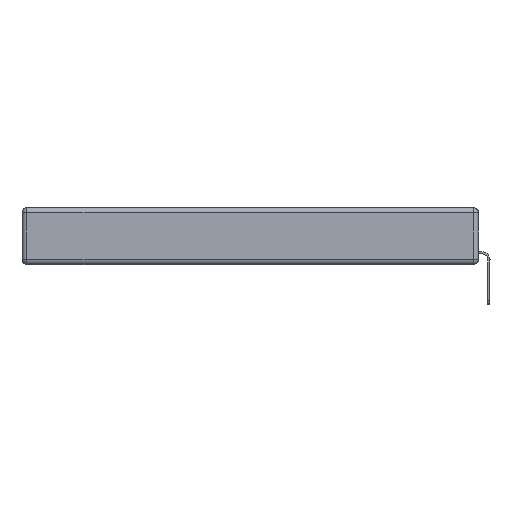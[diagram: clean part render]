
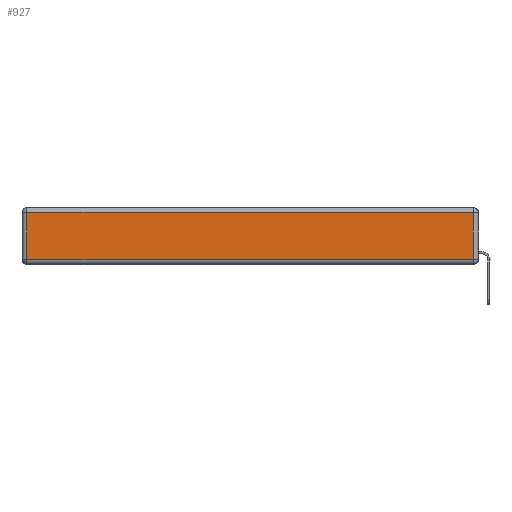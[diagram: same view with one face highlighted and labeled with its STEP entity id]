
A CAD part, left-side view. The second image highlights one B-rep face of the part: STEP entity #927.
In plain terms, the highlighted planar face has unit normal (-1, 0, 0).
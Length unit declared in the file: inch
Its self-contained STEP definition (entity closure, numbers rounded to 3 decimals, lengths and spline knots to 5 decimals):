
#693 = CARTESIAN_POINT ( 'NONE',  ( 0., 0., -0.313 ) ) ;
#814 = DIRECTION ( 'NONE',  ( 0., 0., 1. ) ) ;
#927 = ADVANCED_FACE ( 'NONE', ( #8406 ), #14898, .T. ) ;
#1033 = DIRECTION ( 'NONE',  ( 0., 0., 1. ) ) ;
#1086 = ORIENTED_EDGE ( 'NONE', *, *, #10584, .T. ) ;
#1088 = LINE ( 'NONE', #16699, #4471 ) ;
#1699 = AXIS2_PLACEMENT_3D ( 'NONE', #8491, #7131, #814 ) ;
#2248 = CARTESIAN_POINT ( 'NONE',  ( 0., 2.72, -0.03 ) ) ;
#2648 = CARTESIAN_POINT ( 'NONE',  ( 0., 0.03, -0.03 ) ) ;
#3849 = LINE ( 'NONE', #9047, #4978 ) ;
#4406 = ORIENTED_EDGE ( 'NONE', *, *, #13715, .T. ) ;
#4422 = VECTOR ( 'NONE', #15206, 39.37008 ) ;
#4471 = VECTOR ( 'NONE', #7903, 39.37008 ) ;
#4872 = CARTESIAN_POINT ( 'NONE',  ( 0., 2.72, -0.313 ) ) ;
#4978 = VECTOR ( 'NONE', #1033, 39.37008 ) ;
#5285 = VERTEX_POINT ( 'NONE', #2648 ) ;
#7131 = DIRECTION ( 'NONE',  ( -1., 0., 0. ) ) ;
#7903 = DIRECTION ( 'NONE',  ( 0., 0., -1. ) ) ;
#8406 = FACE_OUTER_BOUND ( 'NONE', #16567, .T. ) ;
#8491 = CARTESIAN_POINT ( 'NONE',  ( 0., 0., -0.343 ) ) ;
#9047 = CARTESIAN_POINT ( 'NONE',  ( 0., 0.03, -0.343 ) ) ;
#10096 = CARTESIAN_POINT ( 'NONE',  ( 0., 0.03, -0.313 ) ) ;
#10444 = EDGE_CURVE ( 'NONE', #5285, #12952, #13930, .T. ) ;
#10560 = VERTEX_POINT ( 'NONE', #4872 ) ;
#10584 = EDGE_CURVE ( 'NONE', #11748, #5285, #3849, .T. ) ;
#11748 = VERTEX_POINT ( 'NONE', #10096 ) ;
#12391 = LINE ( 'NONE', #693, #16205 ) ;
#12469 = DIRECTION ( 'NONE',  ( 0., -1., 0. ) ) ;
#12952 = VERTEX_POINT ( 'NONE', #2248 ) ;
#13715 = EDGE_CURVE ( 'NONE', #12952, #10560, #1088, .T. ) ;
#13724 = ORIENTED_EDGE ( 'NONE', *, *, #14877, .T. ) ;
#13930 = LINE ( 'NONE', #14868, #4422 ) ;
#14400 = ORIENTED_EDGE ( 'NONE', *, *, #10444, .T. ) ;
#14868 = CARTESIAN_POINT ( 'NONE',  ( 0., 2.75, -0.03 ) ) ;
#14877 = EDGE_CURVE ( 'NONE', #10560, #11748, #12391, .T. ) ;
#14898 = PLANE ( 'NONE',  #1699 ) ;
#15206 = DIRECTION ( 'NONE',  ( 0., 1., 0. ) ) ;
#16205 = VECTOR ( 'NONE', #12469, 39.37008 ) ;
#16567 = EDGE_LOOP ( 'NONE', ( #13724, #1086, #14400, #4406 ) ) ;
#16699 = CARTESIAN_POINT ( 'NONE',  ( 0., 2.72, -0.343 ) ) ;
